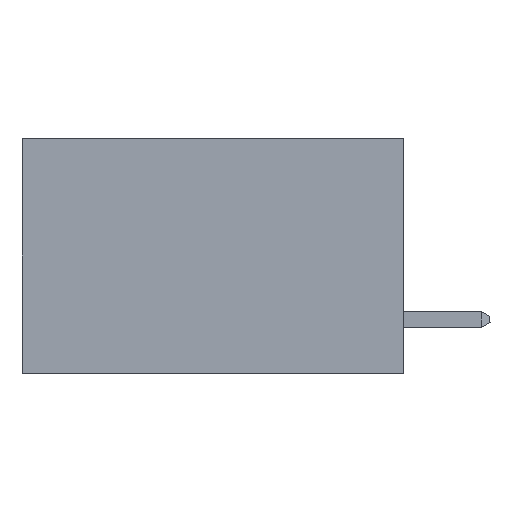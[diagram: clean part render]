
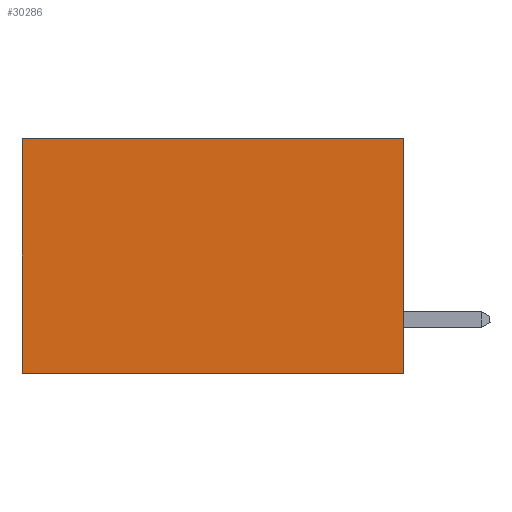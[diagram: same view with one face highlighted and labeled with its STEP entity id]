
A CAD part, left-side view. The second image highlights one B-rep face of the part: STEP entity #30286.
In plain terms, the highlighted planar face has unit normal (-1, 0, 0).
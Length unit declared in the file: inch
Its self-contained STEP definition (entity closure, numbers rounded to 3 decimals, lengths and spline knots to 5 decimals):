
#3111 = CARTESIAN_POINT ( 'NONE',  ( 0.2875, 0.6, -0.37 ) ) ;
#4039 = EDGE_CURVE ( 'NONE', #10631, #23561, #7137, .T. ) ;
#4234 = VERTEX_POINT ( 'NONE', #12141 ) ;
#6725 = DIRECTION ( 'NONE',  ( 0., 0., -1. ) ) ;
#7137 = LINE ( 'NONE', #42511, #37636 ) ;
#7814 = PLANE ( 'NONE',  #30328 ) ;
#7934 = CARTESIAN_POINT ( 'NONE',  ( 0.2875, 0., 0. ) ) ;
#9321 = EDGE_CURVE ( 'NONE', #40944, #10631, #23555, .T. ) ;
#10289 = VECTOR ( 'NONE', #11115, 39.37008 ) ;
#10514 = CARTESIAN_POINT ( 'NONE',  ( 0.2875, 0., 0. ) ) ;
#10631 = VERTEX_POINT ( 'NONE', #39550 ) ;
#11115 = DIRECTION ( 'NONE',  ( 0., 0., -1. ) ) ;
#12141 = CARTESIAN_POINT ( 'NONE',  ( 0.2875, 0.6, 0. ) ) ;
#14227 = EDGE_CURVE ( 'NONE', #40944, #4234, #37431, .T. ) ;
#15603 = ORIENTED_EDGE ( 'NONE', *, *, #9321, .F. ) ;
#16255 = DIRECTION ( 'NONE',  ( 0., 1., 0. ) ) ;
#17522 = FACE_OUTER_BOUND ( 'NONE', #35179, .T. ) ;
#20861 = VECTOR ( 'NONE', #6725, 39.37008 ) ;
#22374 = DIRECTION ( 'NONE',  ( 0., 1., 0. ) ) ;
#23555 = LINE ( 'NONE', #7934, #20861 ) ;
#23561 = VERTEX_POINT ( 'NONE', #3111 ) ;
#25704 = VECTOR ( 'NONE', #16255, 39.37008 ) ;
#27023 = CARTESIAN_POINT ( 'NONE',  ( 0.2875, 0., 0. ) ) ;
#30286 = ADVANCED_FACE ( 'NONE', ( #17522 ), #7814, .F. ) ;
#30328 = AXIS2_PLACEMENT_3D ( 'NONE', #10514, #37982, #41425 ) ;
#31212 = ORIENTED_EDGE ( 'NONE', *, *, #14227, .T. ) ;
#31637 = EDGE_CURVE ( 'NONE', #4234, #23561, #37562, .T. ) ;
#31727 = ORIENTED_EDGE ( 'NONE', *, *, #4039, .F. ) ;
#33990 = ORIENTED_EDGE ( 'NONE', *, *, #31637, .T. ) ;
#34065 = CARTESIAN_POINT ( 'NONE',  ( 0.2875, 0., 0. ) ) ;
#35179 = EDGE_LOOP ( 'NONE', ( #33990, #31727, #15603, #31212 ) ) ;
#37431 = LINE ( 'NONE', #27023, #25704 ) ;
#37562 = LINE ( 'NONE', #42361, #10289 ) ;
#37636 = VECTOR ( 'NONE', #22374, 39.37008 ) ;
#37982 = DIRECTION ( 'NONE',  ( 1., 0., 0. ) ) ;
#39550 = CARTESIAN_POINT ( 'NONE',  ( 0.2875, 0., -0.37 ) ) ;
#40944 = VERTEX_POINT ( 'NONE', #34065 ) ;
#41425 = DIRECTION ( 'NONE',  ( 0., 0., -1. ) ) ;
#42361 = CARTESIAN_POINT ( 'NONE',  ( 0.2875, 0.6, 0. ) ) ;
#42511 = CARTESIAN_POINT ( 'NONE',  ( 0.2875, 0., -0.37 ) ) ;
